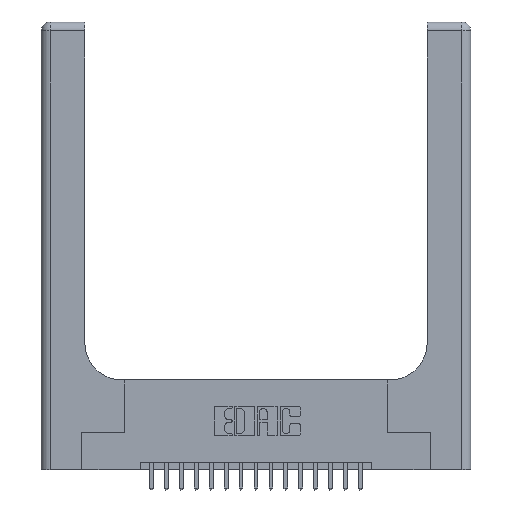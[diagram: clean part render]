
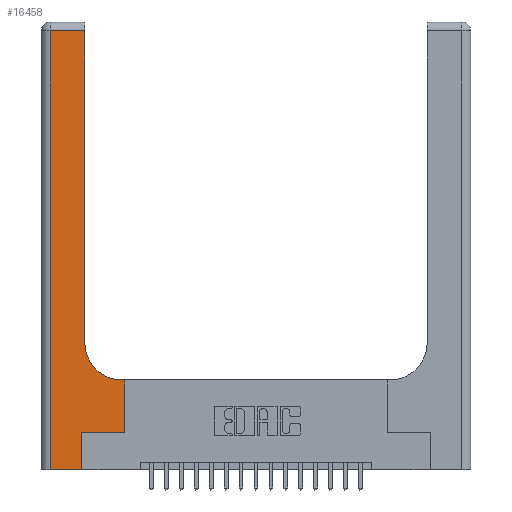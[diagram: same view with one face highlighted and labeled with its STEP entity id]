
A CAD part, top view. The second image highlights one B-rep face of the part: STEP entity #16458.
In plain terms, the highlighted planar face has unit normal (0, 0, 1).
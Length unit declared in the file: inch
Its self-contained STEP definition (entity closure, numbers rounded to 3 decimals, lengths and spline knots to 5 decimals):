
#453 = EDGE_CURVE ( 'NONE', #4361, #12327, #19898, .T. ) ;
#494 = LINE ( 'NONE', #20576, #4756 ) ;
#508 = VERTEX_POINT ( 'NONE', #19900 ) ;
#530 = EDGE_CURVE ( 'NONE', #2404, #6317, #14693, .T. ) ;
#551 = DIRECTION ( 'NONE',  ( 1., 0., 0. ) ) ;
#1413 = CARTESIAN_POINT ( 'NONE',  ( 0.269, 0., 0.37 ) ) ;
#1688 = VERTEX_POINT ( 'NONE', #4339 ) ;
#1733 = LINE ( 'NONE', #12988, #9209 ) ;
#2130 = CARTESIAN_POINT ( 'NONE',  ( 0., 3., 0.37 ) ) ;
#2274 = CARTESIAN_POINT ( 'NONE',  ( 0.2915, 0.85, 0.37 ) ) ;
#2318 = DIRECTION ( 'NONE',  ( 0., 0., -1. ) ) ;
#2404 = VERTEX_POINT ( 'NONE', #18722 ) ;
#2757 = LINE ( 'NONE', #1413, #11214 ) ;
#3886 = ORIENTED_EDGE ( 'NONE', *, *, #19847, .T. ) ;
#3941 = ORIENTED_EDGE ( 'NONE', *, *, #6807, .T. ) ;
#4034 = CARTESIAN_POINT ( 'NONE',  ( 0., 0., 0.37 ) ) ;
#4318 = VERTEX_POINT ( 'NONE', #4358 ) ;
#4339 = CARTESIAN_POINT ( 'NONE',  ( 0.2915, 2.94, 0.37 ) ) ;
#4358 = CARTESIAN_POINT ( 'NONE',  ( 0.269, 0.25, 0.37 ) ) ;
#4361 = VERTEX_POINT ( 'NONE', #15566 ) ;
#4383 = ORIENTED_EDGE ( 'NONE', *, *, #530, .T. ) ;
#4751 = ORIENTED_EDGE ( 'NONE', *, *, #14078, .T. ) ;
#4756 = VECTOR ( 'NONE', #11076, 39.37008 ) ;
#4925 = VECTOR ( 'NONE', #18660, 39.37008 ) ;
#5030 = DIRECTION ( 'NONE',  ( 0., 1., 0. ) ) ;
#5312 = DIRECTION ( 'NONE',  ( -1., 0., 0. ) ) ;
#5429 = LINE ( 'NONE', #17093, #4925 ) ;
#6182 = VECTOR ( 'NONE', #16809, 39.37008 ) ;
#6317 = VERTEX_POINT ( 'NONE', #16371 ) ;
#6457 = CARTESIAN_POINT ( 'NONE',  ( 0.5585, 0.25, 0.37 ) ) ;
#6625 = ORIENTED_EDGE ( 'NONE', *, *, #8505, .T. ) ;
#6708 = EDGE_CURVE ( 'NONE', #6317, #4318, #2757, .T. ) ;
#6807 = EDGE_CURVE ( 'NONE', #16828, #508, #1733, .T. ) ;
#7997 = FACE_OUTER_BOUND ( 'NONE', #20239, .T. ) ;
#8176 = ORIENTED_EDGE ( 'NONE', *, *, #453, .T. ) ;
#8505 = EDGE_CURVE ( 'NONE', #13644, #2404, #16902, .T. ) ;
#9209 = VECTOR ( 'NONE', #5030, 39.37008 ) ;
#9768 = LINE ( 'NONE', #10134, #17765 ) ;
#10134 = CARTESIAN_POINT ( 'NONE',  ( 0.269, 0.25, 0.37 ) ) ;
#10521 = ORIENTED_EDGE ( 'NONE', *, *, #14859, .T. ) ;
#10780 = LINE ( 'NONE', #19521, #18273 ) ;
#11076 = DIRECTION ( 'NONE',  ( 0., 1., 0. ) ) ;
#11214 = VECTOR ( 'NONE', #17380, 39.37008 ) ;
#11855 = CARTESIAN_POINT ( 'NONE',  ( 0.5415, 0.85, 0.37 ) ) ;
#12327 = VERTEX_POINT ( 'NONE', #2274 ) ;
#12649 = VECTOR ( 'NONE', #19164, 39.37008 ) ;
#12988 = CARTESIAN_POINT ( 'NONE',  ( 0.5585, 0.25, 0.37 ) ) ;
#13280 = PLANE ( 'NONE',  #16853 ) ;
#13479 = DIRECTION ( 'NONE',  ( 1., 0., 0. ) ) ;
#13644 = VERTEX_POINT ( 'NONE', #13728 ) ;
#13728 = CARTESIAN_POINT ( 'NONE',  ( 0.06, 2.94, 0.37 ) ) ;
#14078 = EDGE_CURVE ( 'NONE', #508, #4361, #10780, .T. ) ;
#14120 = EDGE_CURVE ( 'NONE', #4318, #16828, #9768, .T. ) ;
#14388 = CARTESIAN_POINT ( 'NONE',  ( 0.06, 3., 0.37 ) ) ;
#14604 = ORIENTED_EDGE ( 'NONE', *, *, #14120, .T. ) ;
#14693 = LINE ( 'NONE', #4034, #6182 ) ;
#14859 = EDGE_CURVE ( 'NONE', #12327, #1688, #494, .T. ) ;
#14875 = DIRECTION ( 'NONE',  ( 0., 0., -1. ) ) ;
#15566 = CARTESIAN_POINT ( 'NONE',  ( 0.5415, 0.6, 0.37 ) ) ;
#16119 = AXIS2_PLACEMENT_3D ( 'NONE', #11855, #2318, #13479 ) ;
#16351 = DIRECTION ( 'NONE',  ( -1., 0., 0. ) ) ;
#16371 = CARTESIAN_POINT ( 'NONE',  ( 0.269, 0., 0.37 ) ) ;
#16458 = ADVANCED_FACE ( 'NONE', ( #7997 ), #13280, .F. ) ;
#16809 = DIRECTION ( 'NONE',  ( 1., 0., 0. ) ) ;
#16828 = VERTEX_POINT ( 'NONE', #6457 ) ;
#16853 = AXIS2_PLACEMENT_3D ( 'NONE', #2130, #14875, #5312 ) ;
#16902 = LINE ( 'NONE', #14388, #12649 ) ;
#17093 = CARTESIAN_POINT ( 'NONE',  ( 0., 2.94, 0.37 ) ) ;
#17380 = DIRECTION ( 'NONE',  ( 0., 1., 0. ) ) ;
#17765 = VECTOR ( 'NONE', #551, 39.37008 ) ;
#18273 = VECTOR ( 'NONE', #16351, 39.37008 ) ;
#18660 = DIRECTION ( 'NONE',  ( -1., 0., 0. ) ) ;
#18722 = CARTESIAN_POINT ( 'NONE',  ( 0.06, 0., 0.37 ) ) ;
#19164 = DIRECTION ( 'NONE',  ( 0., -1., 0. ) ) ;
#19521 = CARTESIAN_POINT ( 'NONE',  ( 0.2915, 0.6, 0.37 ) ) ;
#19847 = EDGE_CURVE ( 'NONE', #1688, #13644, #5429, .T. ) ;
#19898 = CIRCLE ( 'NONE', #16119, 0.25 ) ;
#19900 = CARTESIAN_POINT ( 'NONE',  ( 0.5585, 0.6, 0.37 ) ) ;
#20239 = EDGE_LOOP ( 'NONE', ( #10521, #3886, #6625, #4383, #20257, #14604, #3941, #4751, #8176 ) ) ;
#20257 = ORIENTED_EDGE ( 'NONE', *, *, #6708, .T. ) ;
#20576 = CARTESIAN_POINT ( 'NONE',  ( 0.2915, 3., 0.37 ) ) ;
